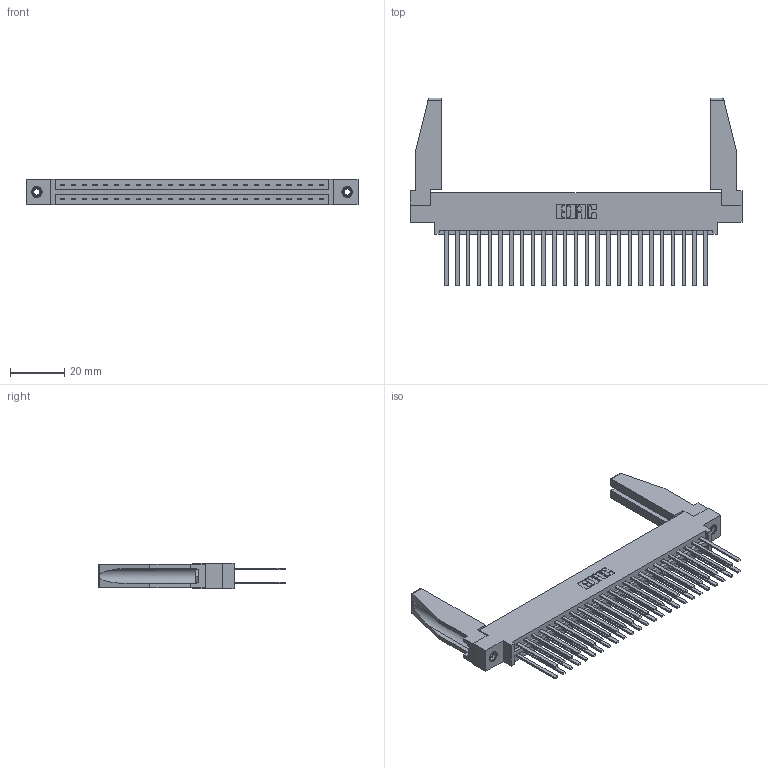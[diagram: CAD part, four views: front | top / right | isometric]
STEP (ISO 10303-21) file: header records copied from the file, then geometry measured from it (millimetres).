
FILE_DESCRIPTION (( 'STEP AP203' ), '1' );
FILE_NAME ('337-050-544-878.STEP', '2019-10-11T17:42:20', ( '' ), ( '' ), 'SwSTEP 2.0', 'SolidWorks 2016', '' );
FILE_SCHEMA (( 'CONFIG_CONTROL_DESIGN' ));
Length unit declared in the file: inch
Products named in the file (5): 307-220-078; 345-292-001_345-293-144; 345-250-001_345-250-001-102; 337-050-544-878; 337 Part_0.170 Offset - 0.156 Dia-TI
Assembly tree (55 placements, depth 2):
  337-050-544-878
    337 Part_0.170 Offset - 0.156 Dia-TI
    345-292-001_345-293-144  x50
    345-250-001_345-250-001-102  x2
    307-220-078  x2
Bounding box: 122.07 x 69.09 x 9.4 mm (x, y, z)
Volume: 17215.4 mm3; surface area: 21010.4 mm2
Topology: 55 solids, 55 shells, 2648 faces, 7803 edges, 5126 vertices
Faces by surface type: plane 1858, cylinder 774, cone 12, torus 4
Entity records: 23970 total; most frequent: CARTESIAN_POINT 4052, ORIENTED_EDGE 3944, DIRECTION 3480, EDGE_CURVE 1972, VECTOR 1810, LINE 1810, VERTEX_POINT 1308, AXIS2_PLACEMENT_3D 835
